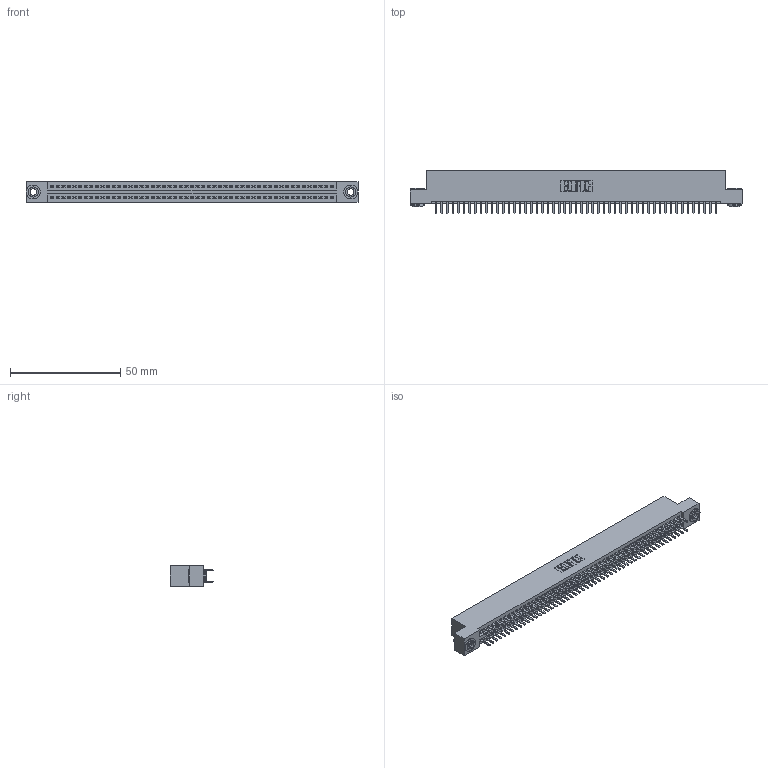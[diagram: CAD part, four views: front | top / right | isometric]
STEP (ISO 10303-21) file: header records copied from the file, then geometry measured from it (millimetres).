
FILE_DESCRIPTION (( 'STEP AP203' ), '1' );
FILE_NAME ('395-102-520-203.STEP', '2018-11-30T04:57:35', ( '' ), ( '' ), 'SwSTEP 2.0', 'SolidWorks 2016', '' );
FILE_SCHEMA (( 'CONFIG_CONTROL_DESIGN' ));
Length unit declared in the file: inch
Products named in the file (4): 345 Part_Flush Mounting Lugs - 0.156 Dia-TH; 345-250-002_345-250-002-102; 345-292-001_345-293-120; 395-102-520-203
Assembly tree (105 placements, depth 2):
  395-102-520-203
    345 Part_Flush Mounting Lugs - 0.156 Dia-TH
    345-292-001_345-293-120  x102
    345-250-002_345-250-002-102  x2
Bounding box: 150.75 x 19.68 x 9.4 mm (x, y, z)
Volume: 14702 mm3; surface area: 22015.9 mm2
Topology: 105 solids, 105 shells, 5672 faces, 16431 edges, 10678 vertices
Faces by surface type: plane 3660, cylinder 2004, cone 8
Entity records: 39568 total; most frequent: CARTESIAN_POINT 6611, ORIENTED_EDGE 6526, DIRECTION 5837, EDGE_CURVE 3263, LINE 2899, VECTOR 2899, VERTEX_POINT 2170, AXIS2_PLACEMENT_3D 1469
